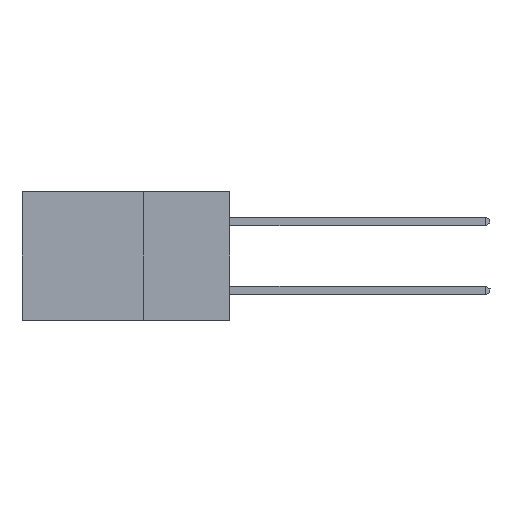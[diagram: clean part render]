
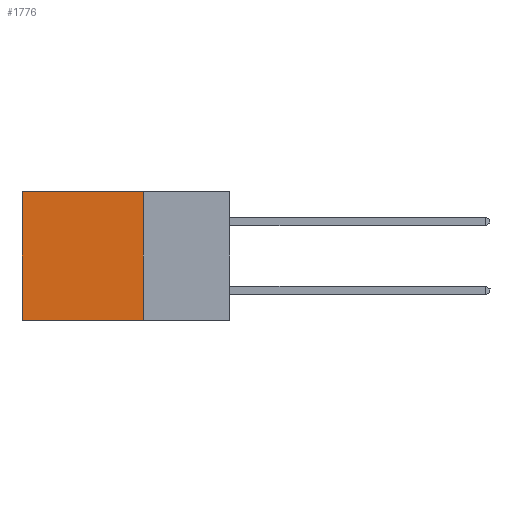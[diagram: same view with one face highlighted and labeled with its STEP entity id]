
A CAD part, left-side view. The second image highlights one B-rep face of the part: STEP entity #1776.
In plain terms, the highlighted planar face has unit normal (-1, 0, 0).
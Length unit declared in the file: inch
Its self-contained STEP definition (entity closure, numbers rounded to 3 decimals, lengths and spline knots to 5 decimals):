
#9 = EDGE_CURVE ( 'NONE', #5980, #1095, #11820, .T. ) ;
#658 = DIRECTION ( 'NONE',  ( 0., 0., -1. ) ) ;
#810 = ORIENTED_EDGE ( 'NONE', *, *, #11189, .F. ) ;
#1020 = CARTESIAN_POINT ( 'NONE',  ( 0.298, 0.25, 0. ) ) ;
#1095 = VERTEX_POINT ( 'NONE', #11873 ) ;
#1156 = LINE ( 'NONE', #1020, #4460 ) ;
#1419 = CARTESIAN_POINT ( 'NONE',  ( 0.298, 0.25, 0. ) ) ;
#1776 = ADVANCED_FACE ( 'NONE', ( #3622 ), #2746, .F. ) ;
#1988 = DIRECTION ( 'NONE',  ( 0., 0., -1. ) ) ;
#2746 = PLANE ( 'NONE',  #3586 ) ;
#2942 = DIRECTION ( 'NONE',  ( 0., 1., 0. ) ) ;
#2981 = CARTESIAN_POINT ( 'NONE',  ( 0.298, 0.6, 0. ) ) ;
#3152 = LINE ( 'NONE', #13313, #5274 ) ;
#3201 = VECTOR ( 'NONE', #2942, 39.37008 ) ;
#3586 = AXIS2_PLACEMENT_3D ( 'NONE', #12224, #7003, #658 ) ;
#3622 = FACE_OUTER_BOUND ( 'NONE', #11033, .T. ) ;
#3685 = LINE ( 'NONE', #6179, #3201 ) ;
#3755 = CARTESIAN_POINT ( 'NONE',  ( 0.298, 0.25, -0.37 ) ) ;
#4460 = VECTOR ( 'NONE', #1988, 39.37008 ) ;
#5206 = VECTOR ( 'NONE', #7372, 39.37008 ) ;
#5274 = VECTOR ( 'NONE', #13266, 39.37008 ) ;
#5941 = VERTEX_POINT ( 'NONE', #3755 ) ;
#5980 = VERTEX_POINT ( 'NONE', #6869 ) ;
#6179 = CARTESIAN_POINT ( 'NONE',  ( 0.298, 0.25, 0. ) ) ;
#6261 = ORIENTED_EDGE ( 'NONE', *, *, #8584, .T. ) ;
#6869 = CARTESIAN_POINT ( 'NONE',  ( 0.298, 0.6, 0. ) ) ;
#7003 = DIRECTION ( 'NONE',  ( 1., 0., 0. ) ) ;
#7372 = DIRECTION ( 'NONE',  ( 0., 0., -1. ) ) ;
#8408 = ORIENTED_EDGE ( 'NONE', *, *, #9585, .F. ) ;
#8584 = EDGE_CURVE ( 'NONE', #12973, #5980, #3685, .T. ) ;
#9585 = EDGE_CURVE ( 'NONE', #12973, #5941, #1156, .T. ) ;
#11033 = EDGE_LOOP ( 'NONE', ( #12960, #810, #8408, #6261 ) ) ;
#11189 = EDGE_CURVE ( 'NONE', #5941, #1095, #3152, .T. ) ;
#11820 = LINE ( 'NONE', #2981, #5206 ) ;
#11873 = CARTESIAN_POINT ( 'NONE',  ( 0.298, 0.6, -0.37 ) ) ;
#12224 = CARTESIAN_POINT ( 'NONE',  ( 0.298, 0.25, 0. ) ) ;
#12960 = ORIENTED_EDGE ( 'NONE', *, *, #9, .T. ) ;
#12973 = VERTEX_POINT ( 'NONE', #1419 ) ;
#13266 = DIRECTION ( 'NONE',  ( 0., 1., 0. ) ) ;
#13313 = CARTESIAN_POINT ( 'NONE',  ( 0.298, 0.25, -0.37 ) ) ;
